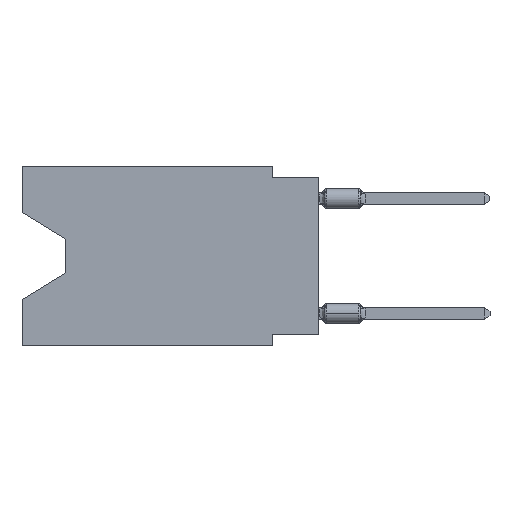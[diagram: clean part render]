
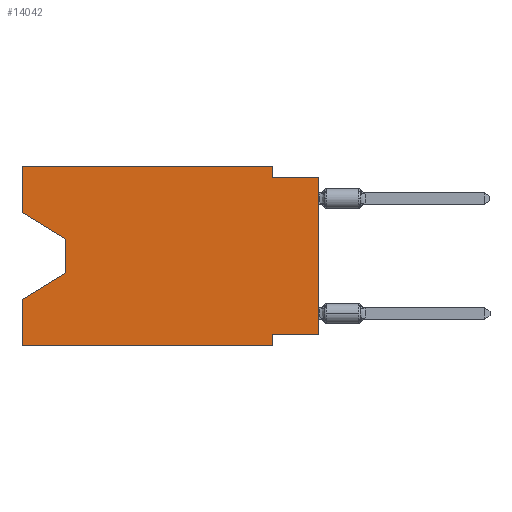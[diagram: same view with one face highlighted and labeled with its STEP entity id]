
A CAD part, left-side view. The second image highlights one B-rep face of the part: STEP entity #14042.
In plain terms, the highlighted planar face has unit normal (-1, 0, 0).
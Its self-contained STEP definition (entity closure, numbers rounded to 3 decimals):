
#104 = VECTOR ( 'NONE', #2377, 1000. ) ;
#244 = ORIENTED_EDGE ( 'NONE', *, *, #10141, .F. ) ;
#492 = VECTOR ( 'NONE', #13120, 1000. ) ;
#508 = LINE ( 'NONE', #10093, #2154 ) ;
#557 = CARTESIAN_POINT ( 'NONE',  ( 0., 16.383, -9.906 ) ) ;
#998 = CARTESIAN_POINT ( 'NONE',  ( 0., 16.383, -2.546 ) ) ;
#1371 = CARTESIAN_POINT ( 'NONE',  ( 0., 0., -9.271 ) ) ;
#1664 = VERTEX_POINT ( 'NONE', #8053 ) ;
#1722 = EDGE_CURVE ( 'NONE', #15718, #5693, #5806, .T. ) ;
#1841 = VERTEX_POINT ( 'NONE', #998 ) ;
#1933 = LINE ( 'NONE', #13010, #8431 ) ;
#2063 = CARTESIAN_POINT ( 'NONE',  ( 0., 16.383, -7.36 ) ) ;
#2131 = EDGE_CURVE ( 'NONE', #15366, #2337, #8309, .T. ) ;
#2154 = VECTOR ( 'NONE', #12724, 1000. ) ;
#2337 = VERTEX_POINT ( 'NONE', #9023 ) ;
#2377 = DIRECTION ( 'NONE',  ( 0., 0.855, -0.519 ) ) ;
#2564 = DIRECTION ( 'NONE',  ( 1., 0., 0. ) ) ;
#2597 = VECTOR ( 'NONE', #15351, 1000. ) ;
#2652 = CARTESIAN_POINT ( 'NONE',  ( 0., 2.54, -9.906 ) ) ;
#2817 = VERTEX_POINT ( 'NONE', #2063 ) ;
#2822 = CARTESIAN_POINT ( 'NONE',  ( 0., 16.383, 0. ) ) ;
#3172 = VECTOR ( 'NONE', #5137, 1000. ) ;
#3554 = VERTEX_POINT ( 'NONE', #12188 ) ;
#3579 = VECTOR ( 'NONE', #6902, 1000. ) ;
#3592 = DIRECTION ( 'NONE',  ( 0., 0., 1. ) ) ;
#3596 = EDGE_CURVE ( 'NONE', #8818, #2817, #8444, .T. ) ;
#3863 = LINE ( 'NONE', #2822, #3172 ) ;
#4222 = EDGE_CURVE ( 'NONE', #1841, #3554, #12947, .T. ) ;
#4466 = CARTESIAN_POINT ( 'NONE',  ( 0., 16.383, 0. ) ) ;
#4520 = EDGE_CURVE ( 'NONE', #7722, #5693, #11260, .T. ) ;
#4913 = VECTOR ( 'NONE', #12610, 1000. ) ;
#5137 = DIRECTION ( 'NONE',  ( 0., 0., 1. ) ) ;
#5693 = VERTEX_POINT ( 'NONE', #2652 ) ;
#5741 = EDGE_CURVE ( 'NONE', #7722, #2817, #3863, .T. ) ;
#5758 = EDGE_CURVE ( 'NONE', #15366, #15718, #10085, .T. ) ;
#5759 = CARTESIAN_POINT ( 'NONE',  ( 0., 13.97, -5.893 ) ) ;
#5806 = LINE ( 'NONE', #11874, #6078 ) ;
#6078 = VECTOR ( 'NONE', #9466, 1000. ) ;
#6447 = ORIENTED_EDGE ( 'NONE', *, *, #10035, .T. ) ;
#6809 = CARTESIAN_POINT ( 'NONE',  ( 0., 2.54, 0. ) ) ;
#6902 = DIRECTION ( 'NONE',  ( 0., -1., 0. ) ) ;
#7067 = CARTESIAN_POINT ( 'NONE',  ( 0., 16.383, 0. ) ) ;
#7291 = ORIENTED_EDGE ( 'NONE', *, *, #1722, .F. ) ;
#7358 = CARTESIAN_POINT ( 'NONE',  ( 0., 16.383, 0. ) ) ;
#7456 = ORIENTED_EDGE ( 'NONE', *, *, #4222, .T. ) ;
#7616 = VECTOR ( 'NONE', #10708, 1000. ) ;
#7722 = VERTEX_POINT ( 'NONE', #11505 ) ;
#8041 = ORIENTED_EDGE ( 'NONE', *, *, #13754, .F. ) ;
#8053 = CARTESIAN_POINT ( 'NONE',  ( 0., 2.54, -0.635 ) ) ;
#8110 = ORIENTED_EDGE ( 'NONE', *, *, #4520, .T. ) ;
#8253 = VECTOR ( 'NONE', #13671, 1000. ) ;
#8309 = LINE ( 'NONE', #15571, #7616 ) ;
#8431 = VECTOR ( 'NONE', #10627, 1000. ) ;
#8444 = LINE ( 'NONE', #13303, #104 ) ;
#8535 = LINE ( 'NONE', #11002, #13523 ) ;
#8557 = FACE_OUTER_BOUND ( 'NONE', #12560, .T. ) ;
#8697 = ORIENTED_EDGE ( 'NONE', *, *, #12592, .F. ) ;
#8818 = VERTEX_POINT ( 'NONE', #5759 ) ;
#9023 = CARTESIAN_POINT ( 'NONE',  ( 0., 0., -0.635 ) ) ;
#9466 = DIRECTION ( 'NONE',  ( 0., 0., -1. ) ) ;
#10035 = EDGE_CURVE ( 'NONE', #3554, #8818, #1933, .T. ) ;
#10074 = AXIS2_PLACEMENT_3D ( 'NONE', #7358, #2564, #13490 ) ;
#10085 = LINE ( 'NONE', #1371, #8253 ) ;
#10093 = CARTESIAN_POINT ( 'NONE',  ( 0., 2.54, 0. ) ) ;
#10141 = EDGE_CURVE ( 'NONE', #1841, #10432, #8535, .T. ) ;
#10250 = ORIENTED_EDGE ( 'NONE', *, *, #5741, .F. ) ;
#10432 = VERTEX_POINT ( 'NONE', #4466 ) ;
#10627 = DIRECTION ( 'NONE',  ( 0., 0., -1. ) ) ;
#10645 = LINE ( 'NONE', #12956, #3579 ) ;
#10652 = ORIENTED_EDGE ( 'NONE', *, *, #2131, .T. ) ;
#10708 = DIRECTION ( 'NONE',  ( 0., 0., 1. ) ) ;
#11002 = CARTESIAN_POINT ( 'NONE',  ( 0., 16.383, 0. ) ) ;
#11065 = EDGE_CURVE ( 'NONE', #10432, #14301, #14317, .T. ) ;
#11260 = LINE ( 'NONE', #557, #4913 ) ;
#11505 = CARTESIAN_POINT ( 'NONE',  ( 0., 16.383, -9.906 ) ) ;
#11544 = ORIENTED_EDGE ( 'NONE', *, *, #5758, .F. ) ;
#11874 = CARTESIAN_POINT ( 'NONE',  ( 0., 2.54, -9.906 ) ) ;
#12151 = ORIENTED_EDGE ( 'NONE', *, *, #3596, .T. ) ;
#12188 = CARTESIAN_POINT ( 'NONE',  ( 0., 13.97, -4.013 ) ) ;
#12560 = EDGE_LOOP ( 'NONE', ( #7456, #6447, #12151, #10250, #8110, #7291, #11544, #10652, #8697, #8041, #13651, #244 ) ) ;
#12592 = EDGE_CURVE ( 'NONE', #1664, #2337, #10645, .T. ) ;
#12610 = DIRECTION ( 'NONE',  ( 0., -1., 0. ) ) ;
#12724 = DIRECTION ( 'NONE',  ( 0., 0., -1. ) ) ;
#12947 = LINE ( 'NONE', #14225, #2597 ) ;
#12956 = CARTESIAN_POINT ( 'NONE',  ( 0., 0., -0.635 ) ) ;
#13010 = CARTESIAN_POINT ( 'NONE',  ( 0., 13.97, -4.013 ) ) ;
#13120 = DIRECTION ( 'NONE',  ( 0., -1., 0. ) ) ;
#13303 = CARTESIAN_POINT ( 'NONE',  ( 0., 13.97, -5.893 ) ) ;
#13416 = PLANE ( 'NONE',  #10074 ) ;
#13490 = DIRECTION ( 'NONE',  ( 0., 0., -1. ) ) ;
#13523 = VECTOR ( 'NONE', #3592, 1000. ) ;
#13651 = ORIENTED_EDGE ( 'NONE', *, *, #11065, .F. ) ;
#13671 = DIRECTION ( 'NONE',  ( 0., 1., 0. ) ) ;
#13754 = EDGE_CURVE ( 'NONE', #14301, #1664, #508, .T. ) ;
#14042 = ADVANCED_FACE ( 'NONE', ( #8557 ), #13416, .F. ) ;
#14225 = CARTESIAN_POINT ( 'NONE',  ( 0., 16.383, -2.546 ) ) ;
#14301 = VERTEX_POINT ( 'NONE', #6809 ) ;
#14317 = LINE ( 'NONE', #7067, #492 ) ;
#14400 = CARTESIAN_POINT ( 'NONE',  ( 0., 2.54, -9.271 ) ) ;
#14496 = CARTESIAN_POINT ( 'NONE',  ( 0., 0., -9.271 ) ) ;
#15351 = DIRECTION ( 'NONE',  ( 0., -0.855, -0.519 ) ) ;
#15366 = VERTEX_POINT ( 'NONE', #14496 ) ;
#15571 = CARTESIAN_POINT ( 'NONE',  ( 0., 0., 0. ) ) ;
#15718 = VERTEX_POINT ( 'NONE', #14400 ) ;
